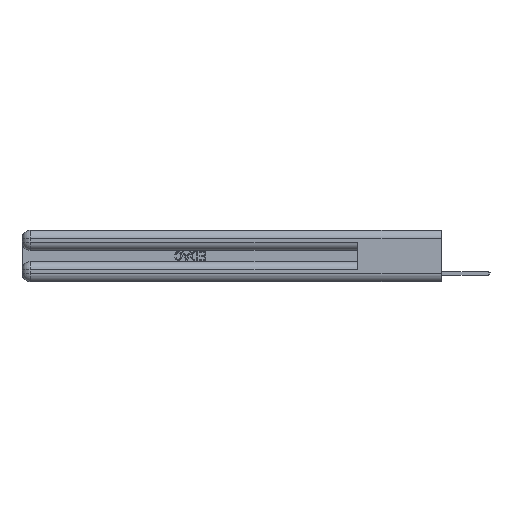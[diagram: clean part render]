
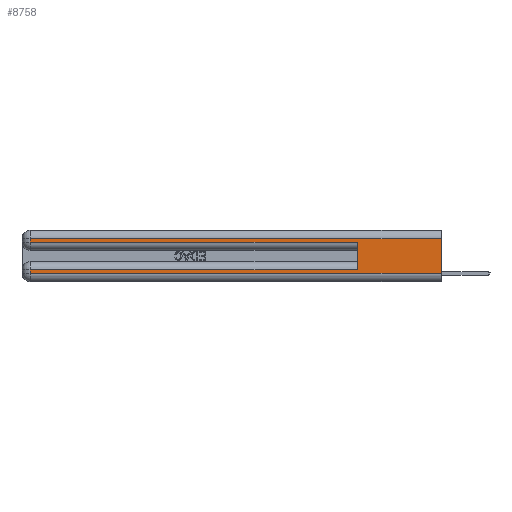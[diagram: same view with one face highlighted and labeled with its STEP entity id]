
A CAD part, left-side view. The second image highlights one B-rep face of the part: STEP entity #8758.
In plain terms, the highlighted planar face has unit normal (-1, 0, 0).
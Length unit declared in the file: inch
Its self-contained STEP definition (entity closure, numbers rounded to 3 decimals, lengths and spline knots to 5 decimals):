
#155 = VECTOR ( 'NONE', #11407, 39.37008 ) ;
#397 = LINE ( 'NONE', #16388, #25195 ) ;
#508 = VERTEX_POINT ( 'NONE', #17582 ) ;
#1145 = VECTOR ( 'NONE', #17150, 39.37008 ) ;
#1282 = CARTESIAN_POINT ( 'NONE',  ( 0., 0., 0.37 ) ) ;
#1467 = CARTESIAN_POINT ( 'NONE',  ( 0., 0., 0.085 ) ) ;
#2154 = EDGE_CURVE ( 'NONE', #7912, #13299, #24803, .T. ) ;
#2305 = VECTOR ( 'NONE', #26623, 39.37008 ) ;
#2555 = VERTEX_POINT ( 'NONE', #8264 ) ;
#3303 = VERTEX_POINT ( 'NONE', #19504 ) ;
#3686 = LINE ( 'NONE', #24101, #6332 ) ;
#3942 = DIRECTION ( 'NONE',  ( 0., 0., -1. ) ) ;
#4653 = DIRECTION ( 'NONE',  ( 0., 1., 0. ) ) ;
#5020 = CARTESIAN_POINT ( 'NONE',  ( 0., 2.94, 0.085 ) ) ;
#5181 = EDGE_CURVE ( 'NONE', #7912, #508, #17333, .T. ) ;
#5728 = CARTESIAN_POINT ( 'NONE',  ( 0., 0.6, 0.085 ) ) ;
#6332 = VECTOR ( 'NONE', #26163, 39.37008 ) ;
#6505 = VERTEX_POINT ( 'NONE', #22294 ) ;
#6634 = EDGE_CURVE ( 'NONE', #17071, #6505, #397, .T. ) ;
#6758 = AXIS2_PLACEMENT_3D ( 'NONE', #1282, #26433, #24473 ) ;
#6782 = VECTOR ( 'NONE', #3942, 39.37008 ) ;
#7569 = EDGE_CURVE ( 'NONE', #13299, #3303, #3686, .T. ) ;
#7912 = VERTEX_POINT ( 'NONE', #24883 ) ;
#8264 = CARTESIAN_POINT ( 'NONE',  ( 0., 0.6, 0.285 ) ) ;
#8758 = ADVANCED_FACE ( 'NONE', ( #9226 ), #19937, .F. ) ;
#8774 = CARTESIAN_POINT ( 'NONE',  ( 0., 0.6, 0.145 ) ) ;
#9181 = VECTOR ( 'NONE', #26387, 39.37008 ) ;
#9226 = FACE_OUTER_BOUND ( 'NONE', #24933, .T. ) ;
#9893 = ORIENTED_EDGE ( 'NONE', *, *, #17120, .T. ) ;
#10355 = DIRECTION ( 'NONE',  ( 0., 0., -1. ) ) ;
#10548 = EDGE_CURVE ( 'NONE', #23132, #17071, #13915, .T. ) ;
#10557 = CARTESIAN_POINT ( 'NONE',  ( 0., 2.94, 0.31 ) ) ;
#10807 = EDGE_CURVE ( 'NONE', #23132, #2555, #23620, .T. ) ;
#10829 = LINE ( 'NONE', #24152, #9181 ) ;
#10902 = ORIENTED_EDGE ( 'NONE', *, *, #5181, .F. ) ;
#11407 = DIRECTION ( 'NONE',  ( 0., -1., 0. ) ) ;
#11672 = ORIENTED_EDGE ( 'NONE', *, *, #10807, .F. ) ;
#13095 = LINE ( 'NONE', #15543, #155 ) ;
#13299 = VERTEX_POINT ( 'NONE', #10557 ) ;
#13915 = LINE ( 'NONE', #1467, #2305 ) ;
#15543 = CARTESIAN_POINT ( 'NONE',  ( 0., 0., 0.285 ) ) ;
#16388 = CARTESIAN_POINT ( 'NONE',  ( 0., 2.94, 0.37 ) ) ;
#16554 = CARTESIAN_POINT ( 'NONE',  ( 0., 0., 0.37 ) ) ;
#17071 = VERTEX_POINT ( 'NONE', #5020 ) ;
#17094 = CARTESIAN_POINT ( 'NONE',  ( 0., 0., 0.31 ) ) ;
#17120 = EDGE_CURVE ( 'NONE', #3303, #2555, #13095, .T. ) ;
#17150 = DIRECTION ( 'NONE',  ( 0., 0., 1. ) ) ;
#17333 = LINE ( 'NONE', #16554, #6782 ) ;
#17582 = CARTESIAN_POINT ( 'NONE',  ( 0., 0., 0.06 ) ) ;
#19504 = CARTESIAN_POINT ( 'NONE',  ( 0., 2.94, 0.285 ) ) ;
#19937 = PLANE ( 'NONE',  #6758 ) ;
#19966 = ORIENTED_EDGE ( 'NONE', *, *, #10548, .T. ) ;
#22294 = CARTESIAN_POINT ( 'NONE',  ( 0., 2.94, 0.06 ) ) ;
#22537 = ORIENTED_EDGE ( 'NONE', *, *, #26898, .T. ) ;
#23132 = VERTEX_POINT ( 'NONE', #5728 ) ;
#23353 = ORIENTED_EDGE ( 'NONE', *, *, #6634, .T. ) ;
#23620 = LINE ( 'NONE', #8774, #1145 ) ;
#24101 = CARTESIAN_POINT ( 'NONE',  ( 0., 2.94, 0.37 ) ) ;
#24152 = CARTESIAN_POINT ( 'NONE',  ( 0., 0., 0.06 ) ) ;
#24473 = DIRECTION ( 'NONE',  ( 0., 0., -1. ) ) ;
#24491 = VECTOR ( 'NONE', #4653, 39.37008 ) ;
#24803 = LINE ( 'NONE', #17094, #24491 ) ;
#24883 = CARTESIAN_POINT ( 'NONE',  ( 0., 0., 0.31 ) ) ;
#24933 = EDGE_LOOP ( 'NONE', ( #10902, #26560, #27069, #9893, #11672, #19966, #23353, #22537 ) ) ;
#25195 = VECTOR ( 'NONE', #10355, 39.37008 ) ;
#26163 = DIRECTION ( 'NONE',  ( 0., 0., -1. ) ) ;
#26387 = DIRECTION ( 'NONE',  ( 0., -1., 0. ) ) ;
#26433 = DIRECTION ( 'NONE',  ( 1., 0., 0. ) ) ;
#26560 = ORIENTED_EDGE ( 'NONE', *, *, #2154, .T. ) ;
#26623 = DIRECTION ( 'NONE',  ( 0., 1., 0. ) ) ;
#26898 = EDGE_CURVE ( 'NONE', #6505, #508, #10829, .T. ) ;
#27069 = ORIENTED_EDGE ( 'NONE', *, *, #7569, .T. ) ;
